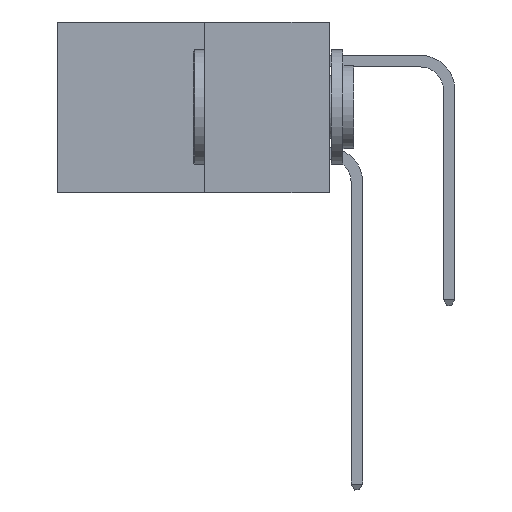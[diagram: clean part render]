
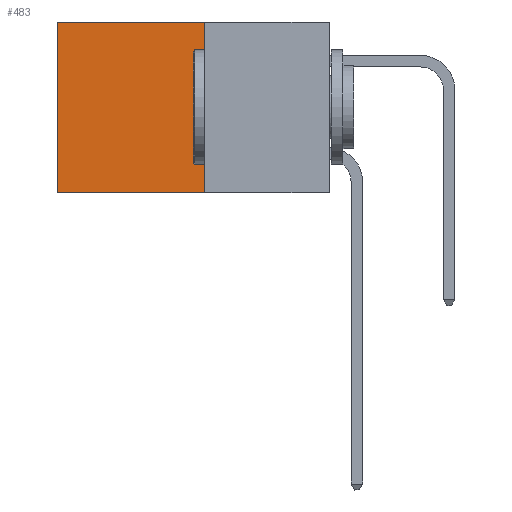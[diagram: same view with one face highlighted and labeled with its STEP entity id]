
A CAD part, left-side view. The second image highlights one B-rep face of the part: STEP entity #483.
In plain terms, the highlighted planar face has unit normal (-1, 0, 0).
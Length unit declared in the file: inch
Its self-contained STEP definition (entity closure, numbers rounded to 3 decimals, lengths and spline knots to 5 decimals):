
#105 = CARTESIAN_POINT ( 'NONE',  ( 0.277, 0.27, -0.37 ) ) ;
#483 = ADVANCED_FACE ( 'NONE', ( #15771 ), #13359, .F. ) ;
#490 = EDGE_CURVE ( 'NONE', #7911, #10247, #3288, .T. ) ;
#3263 = DIRECTION ( 'NONE',  ( 0., 1., 0. ) ) ;
#3288 = LINE ( 'NONE', #105, #12170 ) ;
#3524 = CARTESIAN_POINT ( 'NONE',  ( 0.277, 0.59, -0.37 ) ) ;
#3587 = ORIENTED_EDGE ( 'NONE', *, *, #5053, .T. ) ;
#4529 = ORIENTED_EDGE ( 'NONE', *, *, #19368, .F. ) ;
#5053 = EDGE_CURVE ( 'NONE', #7911, #5364, #15498, .T. ) ;
#5095 = DIRECTION ( 'NONE',  ( 0., 0., -1. ) ) ;
#5364 = VERTEX_POINT ( 'NONE', #18017 ) ;
#7204 = VECTOR ( 'NONE', #14949, 39.37008 ) ;
#7666 = VECTOR ( 'NONE', #3263, 39.37008 ) ;
#7794 = EDGE_LOOP ( 'NONE', ( #13141, #4529, #11209, #3587 ) ) ;
#7911 = VERTEX_POINT ( 'NONE', #19208 ) ;
#8144 = LINE ( 'NONE', #3524, #11321 ) ;
#8830 = VERTEX_POINT ( 'NONE', #10723 ) ;
#9526 = CARTESIAN_POINT ( 'NONE',  ( 0.277, 0.27, -0.37 ) ) ;
#10247 = VERTEX_POINT ( 'NONE', #10931 ) ;
#10723 = CARTESIAN_POINT ( 'NONE',  ( 0.277, 0.59, -0.37 ) ) ;
#10931 = CARTESIAN_POINT ( 'NONE',  ( 0.277, 0.27, -0.37 ) ) ;
#11209 = ORIENTED_EDGE ( 'NONE', *, *, #490, .F. ) ;
#11321 = VECTOR ( 'NONE', #5095, 39.37008 ) ;
#12170 = VECTOR ( 'NONE', #12701, 39.37008 ) ;
#12701 = DIRECTION ( 'NONE',  ( 0., 0., -1. ) ) ;
#13141 = ORIENTED_EDGE ( 'NONE', *, *, #15556, .T. ) ;
#13359 = PLANE ( 'NONE',  #19113 ) ;
#14280 = CARTESIAN_POINT ( 'NONE',  ( 0.277, 0.27, -0.37 ) ) ;
#14604 = CARTESIAN_POINT ( 'NONE',  ( 0.277, 0.27, 0. ) ) ;
#14949 = DIRECTION ( 'NONE',  ( 0., 1., 0. ) ) ;
#15307 = DIRECTION ( 'NONE',  ( 0., 0., -1. ) ) ;
#15498 = LINE ( 'NONE', #14604, #7204 ) ;
#15556 = EDGE_CURVE ( 'NONE', #5364, #8830, #8144, .T. ) ;
#15771 = FACE_OUTER_BOUND ( 'NONE', #7794, .T. ) ;
#16395 = LINE ( 'NONE', #9526, #7666 ) ;
#18017 = CARTESIAN_POINT ( 'NONE',  ( 0.277, 0.59, 0. ) ) ;
#18355 = DIRECTION ( 'NONE',  ( 1., 0., 0. ) ) ;
#19113 = AXIS2_PLACEMENT_3D ( 'NONE', #14280, #18355, #15307 ) ;
#19208 = CARTESIAN_POINT ( 'NONE',  ( 0.277, 0.27, 0. ) ) ;
#19368 = EDGE_CURVE ( 'NONE', #10247, #8830, #16395, .T. ) ;
